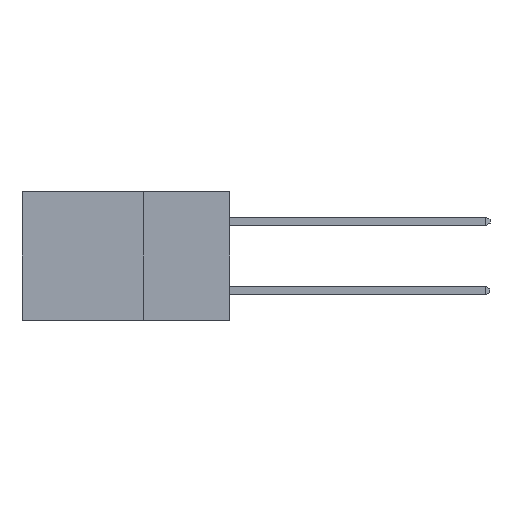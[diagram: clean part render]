
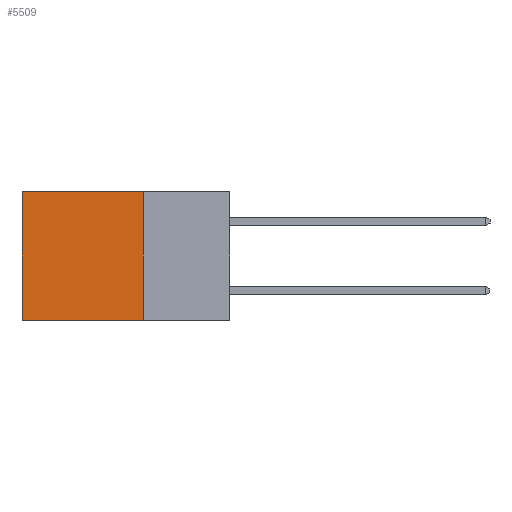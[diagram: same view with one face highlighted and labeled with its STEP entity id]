
A CAD part, left-side view. The second image highlights one B-rep face of the part: STEP entity #5509.
In plain terms, the highlighted planar face has unit normal (-1, 0, 0).
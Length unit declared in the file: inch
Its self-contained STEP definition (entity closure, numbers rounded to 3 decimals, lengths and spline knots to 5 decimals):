
#635 = AXIS2_PLACEMENT_3D ( 'NONE', #18602, #20909, #6698 ) ;
#1291 = VERTEX_POINT ( 'NONE', #13581 ) ;
#1923 = PLANE ( 'NONE',  #635 ) ;
#1961 = EDGE_LOOP ( 'NONE', ( #8590, #25082, #17537, #13512 ) ) ;
#3306 = EDGE_CURVE ( 'NONE', #1291, #15734, #14850, .T. ) ;
#4397 = DIRECTION ( 'NONE',  ( 0., 1., 0. ) ) ;
#5509 = ADVANCED_FACE ( 'NONE', ( #27159 ), #1923, .F. ) ;
#6698 = DIRECTION ( 'NONE',  ( 0., 0., -1. ) ) ;
#7158 = EDGE_CURVE ( 'NONE', #15734, #18470, #14255, .T. ) ;
#7901 = VECTOR ( 'NONE', #15303, 39.37008 ) ;
#8500 = VECTOR ( 'NONE', #12346, 39.37008 ) ;
#8590 = ORIENTED_EDGE ( 'NONE', *, *, #18359, .T. ) ;
#9131 = CARTESIAN_POINT ( 'NONE',  ( 0.298, 0.25, -0.37 ) ) ;
#9364 = CARTESIAN_POINT ( 'NONE',  ( 0.298, 0.6, 0. ) ) ;
#9963 = VECTOR ( 'NONE', #4397, 39.37008 ) ;
#10513 = CARTESIAN_POINT ( 'NONE',  ( 0.298, 0.25, -0.37 ) ) ;
#10725 = VERTEX_POINT ( 'NONE', #17961 ) ;
#12346 = DIRECTION ( 'NONE',  ( 0., 0., -1. ) ) ;
#13512 = ORIENTED_EDGE ( 'NONE', *, *, #29755, .T. ) ;
#13581 = CARTESIAN_POINT ( 'NONE',  ( 0.298, 0.25, 0. ) ) ;
#14255 = LINE ( 'NONE', #10513, #7901 ) ;
#14476 = LINE ( 'NONE', #9364, #26918 ) ;
#14850 = LINE ( 'NONE', #19375, #8500 ) ;
#15303 = DIRECTION ( 'NONE',  ( 0., 1., 0. ) ) ;
#15734 = VERTEX_POINT ( 'NONE', #9131 ) ;
#16295 = LINE ( 'NONE', #23200, #9963 ) ;
#17394 = CARTESIAN_POINT ( 'NONE',  ( 0.298, 0.6, -0.37 ) ) ;
#17537 = ORIENTED_EDGE ( 'NONE', *, *, #3306, .F. ) ;
#17961 = CARTESIAN_POINT ( 'NONE',  ( 0.298, 0.6, 0. ) ) ;
#18359 = EDGE_CURVE ( 'NONE', #10725, #18470, #14476, .T. ) ;
#18470 = VERTEX_POINT ( 'NONE', #17394 ) ;
#18602 = CARTESIAN_POINT ( 'NONE',  ( 0.298, 0.25, 0. ) ) ;
#19375 = CARTESIAN_POINT ( 'NONE',  ( 0.298, 0.25, 0. ) ) ;
#20909 = DIRECTION ( 'NONE',  ( 1., 0., 0. ) ) ;
#23200 = CARTESIAN_POINT ( 'NONE',  ( 0.298, 0.25, 0. ) ) ;
#23548 = DIRECTION ( 'NONE',  ( 0., 0., -1. ) ) ;
#25082 = ORIENTED_EDGE ( 'NONE', *, *, #7158, .F. ) ;
#26918 = VECTOR ( 'NONE', #23548, 39.37008 ) ;
#27159 = FACE_OUTER_BOUND ( 'NONE', #1961, .T. ) ;
#29755 = EDGE_CURVE ( 'NONE', #1291, #10725, #16295, .T. ) ;
